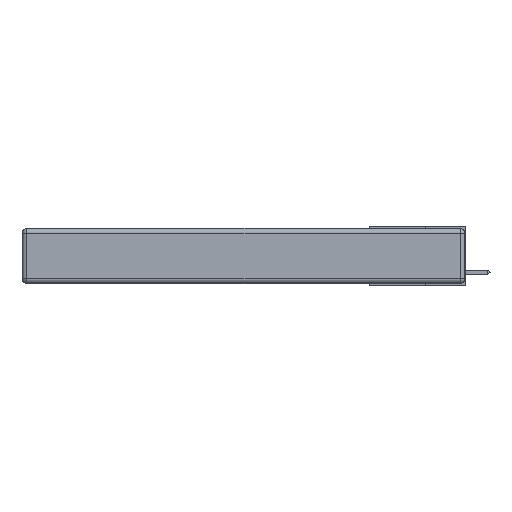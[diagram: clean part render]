
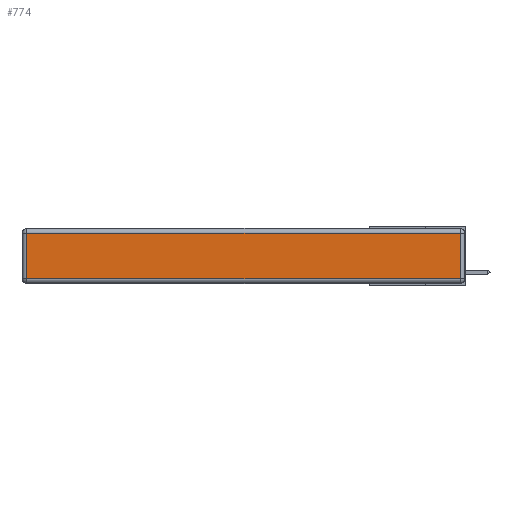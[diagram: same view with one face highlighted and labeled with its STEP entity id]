
A CAD part, left-side view. The second image highlights one B-rep face of the part: STEP entity #774.
In plain terms, the highlighted planar face has unit normal (-1, 0, 0).
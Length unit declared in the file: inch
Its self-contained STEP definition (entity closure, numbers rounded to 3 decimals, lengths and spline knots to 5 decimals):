
#355 = VERTEX_POINT ( 'NONE', #6358 ) ;
#474 = EDGE_LOOP ( 'NONE', ( #1570, #8736, #8894, #10459 ) ) ;
#510 = CARTESIAN_POINT ( 'NONE',  ( 0., 0., -0.313 ) ) ;
#615 = CARTESIAN_POINT ( 'NONE',  ( 0., 2.72, -0.313 ) ) ;
#641 = DIRECTION ( 'NONE',  ( -1., 0., 0. ) ) ;
#774 = ADVANCED_FACE ( 'NONE', ( #15355 ), #8618, .T. ) ;
#1570 = ORIENTED_EDGE ( 'NONE', *, *, #2682, .T. ) ;
#2682 = EDGE_CURVE ( 'NONE', #16144, #10670, #12443, .T. ) ;
#3343 = LINE ( 'NONE', #13063, #17529 ) ;
#3956 = CARTESIAN_POINT ( 'NONE',  ( 0., 2.72, -0.343 ) ) ;
#4029 = CARTESIAN_POINT ( 'NONE',  ( 0., 0.03, -0.313 ) ) ;
#4289 = VERTEX_POINT ( 'NONE', #14173 ) ;
#4718 = DIRECTION ( 'NONE',  ( 0., -1., 0. ) ) ;
#4914 = DIRECTION ( 'NONE',  ( 0., 1., 0. ) ) ;
#6189 = DIRECTION ( 'NONE',  ( 0., 0., 1. ) ) ;
#6358 = CARTESIAN_POINT ( 'NONE',  ( 0., 0.03, -0.03 ) ) ;
#7290 = AXIS2_PLACEMENT_3D ( 'NONE', #13325, #641, #15881 ) ;
#7858 = EDGE_CURVE ( 'NONE', #355, #4289, #8830, .T. ) ;
#7900 = LINE ( 'NONE', #3956, #14452 ) ;
#8618 = PLANE ( 'NONE',  #7290 ) ;
#8736 = ORIENTED_EDGE ( 'NONE', *, *, #15526, .T. ) ;
#8830 = LINE ( 'NONE', #11938, #12973 ) ;
#8894 = ORIENTED_EDGE ( 'NONE', *, *, #7858, .T. ) ;
#10459 = ORIENTED_EDGE ( 'NONE', *, *, #17763, .T. ) ;
#10500 = VECTOR ( 'NONE', #4718, 39.37008 ) ;
#10670 = VERTEX_POINT ( 'NONE', #4029 ) ;
#11938 = CARTESIAN_POINT ( 'NONE',  ( 0., 2.75, -0.03 ) ) ;
#12443 = LINE ( 'NONE', #510, #10500 ) ;
#12973 = VECTOR ( 'NONE', #4914, 39.37008 ) ;
#13063 = CARTESIAN_POINT ( 'NONE',  ( 0., 0.03, -0.343 ) ) ;
#13325 = CARTESIAN_POINT ( 'NONE',  ( 0., 0., -0.343 ) ) ;
#13740 = DIRECTION ( 'NONE',  ( 0., 0., -1. ) ) ;
#14173 = CARTESIAN_POINT ( 'NONE',  ( 0., 2.72, -0.03 ) ) ;
#14452 = VECTOR ( 'NONE', #13740, 39.37008 ) ;
#15355 = FACE_OUTER_BOUND ( 'NONE', #474, .T. ) ;
#15526 = EDGE_CURVE ( 'NONE', #10670, #355, #3343, .T. ) ;
#15881 = DIRECTION ( 'NONE',  ( 0., 0., 1. ) ) ;
#16144 = VERTEX_POINT ( 'NONE', #615 ) ;
#17529 = VECTOR ( 'NONE', #6189, 39.37008 ) ;
#17763 = EDGE_CURVE ( 'NONE', #4289, #16144, #7900, .T. ) ;
